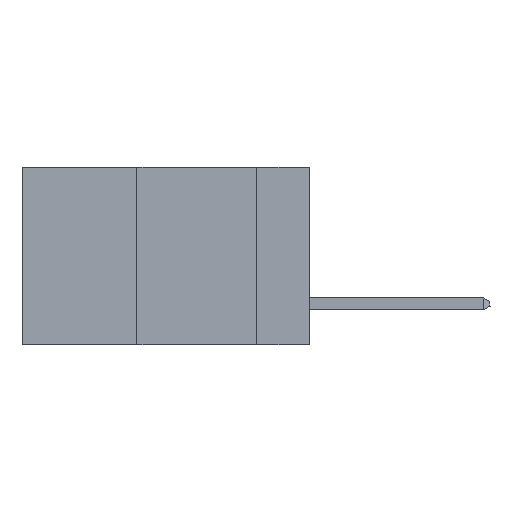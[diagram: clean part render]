
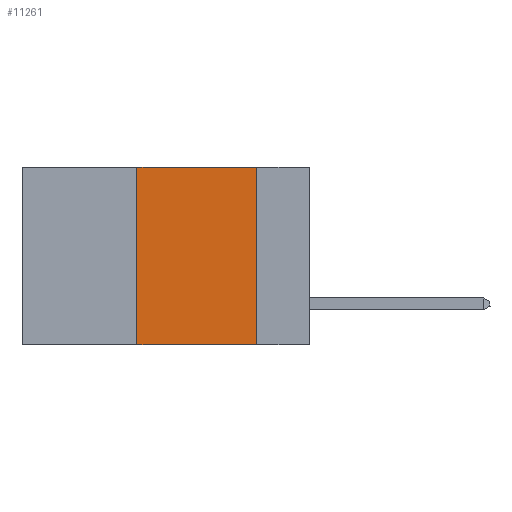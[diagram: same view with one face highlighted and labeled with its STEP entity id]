
A CAD part, left-side view. The second image highlights one B-rep face of the part: STEP entity #11261.
In plain terms, the highlighted planar face has unit normal (-1, 0, 0).
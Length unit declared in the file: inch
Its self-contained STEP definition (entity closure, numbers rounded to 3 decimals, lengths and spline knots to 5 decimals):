
#653 = LINE ( 'NONE', #30850, #13804 ) ;
#4269 = ORIENTED_EDGE ( 'NONE', *, *, #24447, .F. ) ;
#4942 = LINE ( 'NONE', #40250, #6765 ) ;
#5765 = EDGE_CURVE ( 'NONE', #18417, #41830, #12253, .T. ) ;
#6765 = VECTOR ( 'NONE', #17278, 39.37008 ) ;
#7803 = ORIENTED_EDGE ( 'NONE', *, *, #20432, .F. ) ;
#9219 = EDGE_LOOP ( 'NONE', ( #4269, #7803, #47007, #32392 ) ) ;
#11261 = ADVANCED_FACE ( 'NONE', ( #44536 ), #44941, .F. ) ;
#11707 = CARTESIAN_POINT ( 'NONE',  ( 0., 0.11, 0. ) ) ;
#12253 = LINE ( 'NONE', #40003, #18816 ) ;
#12350 = DIRECTION ( 'NONE',  ( 0., -1., 0. ) ) ;
#13779 = CARTESIAN_POINT ( 'NONE',  ( 0., 0.36, 0. ) ) ;
#13804 = VECTOR ( 'NONE', #12350, 39.37008 ) ;
#17278 = DIRECTION ( 'NONE',  ( 0., -1., 0. ) ) ;
#18417 = VERTEX_POINT ( 'NONE', #44127 ) ;
#18816 = VECTOR ( 'NONE', #35687, 39.37008 ) ;
#20432 = EDGE_CURVE ( 'NONE', #41830, #26591, #4942, .T. ) ;
#22380 = CARTESIAN_POINT ( 'NONE',  ( 0., 0.6, 0. ) ) ;
#24447 = EDGE_CURVE ( 'NONE', #26591, #49129, #28946, .T. ) ;
#26591 = VERTEX_POINT ( 'NONE', #44576 ) ;
#28946 = LINE ( 'NONE', #11707, #39130 ) ;
#30850 = CARTESIAN_POINT ( 'NONE',  ( 0., 0.6, -0.37 ) ) ;
#32392 = ORIENTED_EDGE ( 'NONE', *, *, #47944, .T. ) ;
#33422 = DIRECTION ( 'NONE',  ( 1., 0., 0. ) ) ;
#33772 = DIRECTION ( 'NONE',  ( 0., 0., -1. ) ) ;
#34858 = AXIS2_PLACEMENT_3D ( 'NONE', #22380, #33422, #33772 ) ;
#35687 = DIRECTION ( 'NONE',  ( 0., 0., 1. ) ) ;
#39130 = VECTOR ( 'NONE', #46223, 39.37008 ) ;
#40003 = CARTESIAN_POINT ( 'NONE',  ( 0., 0.36, 0. ) ) ;
#40250 = CARTESIAN_POINT ( 'NONE',  ( 0., 0.6, 0. ) ) ;
#41830 = VERTEX_POINT ( 'NONE', #13779 ) ;
#44108 = CARTESIAN_POINT ( 'NONE',  ( 0., 0.11, -0.37 ) ) ;
#44127 = CARTESIAN_POINT ( 'NONE',  ( 0., 0.36, -0.37 ) ) ;
#44536 = FACE_OUTER_BOUND ( 'NONE', #9219, .T. ) ;
#44576 = CARTESIAN_POINT ( 'NONE',  ( 0., 0.11, 0. ) ) ;
#44941 = PLANE ( 'NONE',  #34858 ) ;
#46223 = DIRECTION ( 'NONE',  ( 0., 0., -1. ) ) ;
#47007 = ORIENTED_EDGE ( 'NONE', *, *, #5765, .F. ) ;
#47944 = EDGE_CURVE ( 'NONE', #18417, #49129, #653, .T. ) ;
#49129 = VERTEX_POINT ( 'NONE', #44108 ) ;
